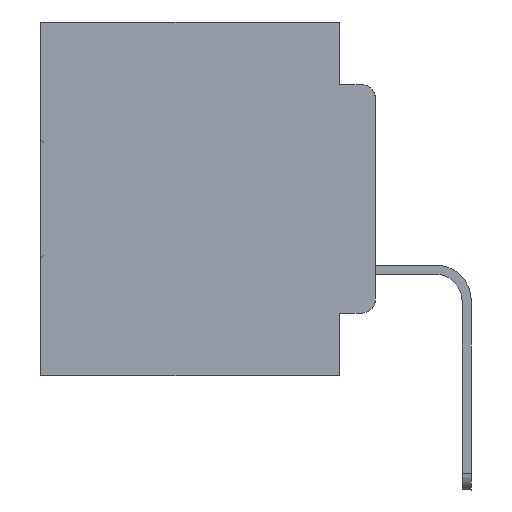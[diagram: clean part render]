
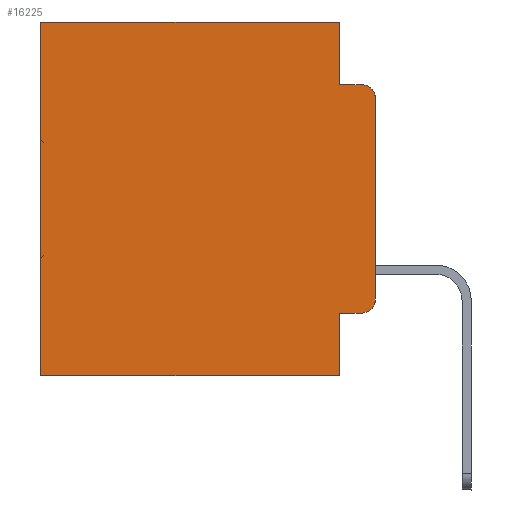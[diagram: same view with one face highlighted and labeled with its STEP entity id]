
A CAD part, left-side view. The second image highlights one B-rep face of the part: STEP entity #16225.
In plain terms, the highlighted planar face has unit normal (-1, 0, 0).
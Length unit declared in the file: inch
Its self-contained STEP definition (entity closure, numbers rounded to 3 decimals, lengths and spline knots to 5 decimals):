
#1254 = CARTESIAN_POINT ( 'NONE',  ( 0.298, 0.473, 0. ) ) ;
#1556 = CIRCLE ( 'NONE', #14137, 0.02 ) ;
#1566 = ORIENTED_EDGE ( 'NONE', *, *, #22731, .F. ) ;
#2893 = CARTESIAN_POINT ( 'NONE',  ( 0.298, 0.051, 0. ) ) ;
#3278 = VERTEX_POINT ( 'NONE', #9668 ) ;
#3466 = DIRECTION ( 'NONE',  ( 0., 0., -1. ) ) ;
#3491 = CARTESIAN_POINT ( 'NONE',  ( 0.298, 0.051, -0.0885 ) ) ;
#3757 = LINE ( 'NONE', #16805, #20361 ) ;
#3810 = VERTEX_POINT ( 'NONE', #14933 ) ;
#4115 = ORIENTED_EDGE ( 'NONE', *, *, #21251, .F. ) ;
#4184 = CARTESIAN_POINT ( 'NONE',  ( 0.298, 0., -0.5 ) ) ;
#4531 = VERTEX_POINT ( 'NONE', #16165 ) ;
#4800 = AXIS2_PLACEMENT_3D ( 'NONE', #22080, #14043, #32391 ) ;
#5301 = LINE ( 'NONE', #13913, #17099 ) ;
#5460 = CARTESIAN_POINT ( 'NONE',  ( 0.298, 0.051, 0. ) ) ;
#5491 = CIRCLE ( 'NONE', #7449, 0.02 ) ;
#7086 = VECTOR ( 'NONE', #21666, 39.37008 ) ;
#7166 = VECTOR ( 'NONE', #11859, 39.37008 ) ;
#7169 = EDGE_CURVE ( 'NONE', #28561, #4531, #31168, .T. ) ;
#7449 = AXIS2_PLACEMENT_3D ( 'NONE', #10569, #18727, #21316 ) ;
#8154 = DIRECTION ( 'NONE',  ( 0., 0., -1. ) ) ;
#8381 = LINE ( 'NONE', #32813, #7166 ) ;
#8784 = CARTESIAN_POINT ( 'NONE',  ( 0.298, 0., -0.3915 ) ) ;
#8978 = PLANE ( 'NONE',  #4800 ) ;
#9665 = LINE ( 'NONE', #15185, #27517 ) ;
#9668 = CARTESIAN_POINT ( 'NONE',  ( 0.298, 0.02, -0.4115 ) ) ;
#10163 = ORIENTED_EDGE ( 'NONE', *, *, #19090, .T. ) ;
#10268 = EDGE_LOOP ( 'NONE', ( #32345, #18417, #1566, #4115, #10540, #31161, #29730, #12635, #10163, #26665 ) ) ;
#10540 = ORIENTED_EDGE ( 'NONE', *, *, #30333, .T. ) ;
#10569 = CARTESIAN_POINT ( 'NONE',  ( 0.298, 0.02, -0.3915 ) ) ;
#11016 = LINE ( 'NONE', #25245, #30481 ) ;
#11797 = CARTESIAN_POINT ( 'NONE',  ( 0.298, 0.02, -0.1085 ) ) ;
#11859 = DIRECTION ( 'NONE',  ( 0., -1., 0. ) ) ;
#12635 = ORIENTED_EDGE ( 'NONE', *, *, #15140, .F. ) ;
#13913 = CARTESIAN_POINT ( 'NONE',  ( 0.298, 0.473, 0. ) ) ;
#13970 = LINE ( 'NONE', #29491, #7086 ) ;
#14043 = DIRECTION ( 'NONE',  ( 1., 0., 0. ) ) ;
#14137 = AXIS2_PLACEMENT_3D ( 'NONE', #11797, #19398, #19717 ) ;
#14933 = CARTESIAN_POINT ( 'NONE',  ( 0.298, 0.02, -0.0885 ) ) ;
#15011 = CARTESIAN_POINT ( 'NONE',  ( 0.298, 0., -0.1085 ) ) ;
#15140 = EDGE_CURVE ( 'NONE', #25811, #28561, #22677, .T. ) ;
#15185 = CARTESIAN_POINT ( 'NONE',  ( 0.298, 0.051, 0. ) ) ;
#16165 = CARTESIAN_POINT ( 'NONE',  ( 0.298, 0.473, -0.5 ) ) ;
#16216 = VERTEX_POINT ( 'NONE', #3491 ) ;
#16225 = ADVANCED_FACE ( 'NONE', ( #18188 ), #8978, .F. ) ;
#16805 = CARTESIAN_POINT ( 'NONE',  ( 0.298, 0., 0. ) ) ;
#17099 = VECTOR ( 'NONE', #3466, 39.37008 ) ;
#17313 = EDGE_CURVE ( 'NONE', #3278, #19053, #5491, .T. ) ;
#17807 = DIRECTION ( 'NONE',  ( 0., 0., -1. ) ) ;
#18188 = FACE_OUTER_BOUND ( 'NONE', #10268, .T. ) ;
#18417 = ORIENTED_EDGE ( 'NONE', *, *, #26735, .T. ) ;
#18727 = DIRECTION ( 'NONE',  ( -1., 0., 0. ) ) ;
#19053 = VERTEX_POINT ( 'NONE', #8784 ) ;
#19090 = EDGE_CURVE ( 'NONE', #25811, #3278, #13970, .T. ) ;
#19275 = DIRECTION ( 'NONE',  ( 0., 1., 0. ) ) ;
#19398 = DIRECTION ( 'NONE',  ( -1., 0., 0. ) ) ;
#19717 = DIRECTION ( 'NONE',  ( 0., 0., -1. ) ) ;
#20361 = VECTOR ( 'NONE', #19275, 39.37008 ) ;
#21251 = EDGE_CURVE ( 'NONE', #23616, #16216, #9665, .T. ) ;
#21316 = DIRECTION ( 'NONE',  ( 0., 0., -1. ) ) ;
#21666 = DIRECTION ( 'NONE',  ( 0., -1., 0. ) ) ;
#22080 = CARTESIAN_POINT ( 'NONE',  ( 0.298, 0., 0. ) ) ;
#22677 = LINE ( 'NONE', #2893, #25951 ) ;
#22731 = EDGE_CURVE ( 'NONE', #16216, #3810, #8381, .T. ) ;
#22779 = VERTEX_POINT ( 'NONE', #15011 ) ;
#23473 = VECTOR ( 'NONE', #30348, 39.37008 ) ;
#23616 = VERTEX_POINT ( 'NONE', #5460 ) ;
#25116 = EDGE_CURVE ( 'NONE', #22779, #19053, #11016, .T. ) ;
#25245 = CARTESIAN_POINT ( 'NONE',  ( 0.298, 0., 0. ) ) ;
#25470 = DIRECTION ( 'NONE',  ( 0., 0., -1. ) ) ;
#25560 = EDGE_CURVE ( 'NONE', #27952, #4531, #5301, .T. ) ;
#25650 = CARTESIAN_POINT ( 'NONE',  ( 0.298, 0.051, -0.4115 ) ) ;
#25811 = VERTEX_POINT ( 'NONE', #25650 ) ;
#25951 = VECTOR ( 'NONE', #8154, 39.37008 ) ;
#26665 = ORIENTED_EDGE ( 'NONE', *, *, #17313, .T. ) ;
#26735 = EDGE_CURVE ( 'NONE', #22779, #3810, #1556, .T. ) ;
#27517 = VECTOR ( 'NONE', #17807, 39.37008 ) ;
#27952 = VERTEX_POINT ( 'NONE', #1254 ) ;
#28561 = VERTEX_POINT ( 'NONE', #29371 ) ;
#29371 = CARTESIAN_POINT ( 'NONE',  ( 0.298, 0.051, -0.5 ) ) ;
#29491 = CARTESIAN_POINT ( 'NONE',  ( 0.298, 0.051, -0.4115 ) ) ;
#29730 = ORIENTED_EDGE ( 'NONE', *, *, #7169, .F. ) ;
#30333 = EDGE_CURVE ( 'NONE', #23616, #27952, #3757, .T. ) ;
#30348 = DIRECTION ( 'NONE',  ( 0., 1., 0. ) ) ;
#30481 = VECTOR ( 'NONE', #25470, 39.37008 ) ;
#31161 = ORIENTED_EDGE ( 'NONE', *, *, #25560, .T. ) ;
#31168 = LINE ( 'NONE', #4184, #23473 ) ;
#32345 = ORIENTED_EDGE ( 'NONE', *, *, #25116, .F. ) ;
#32391 = DIRECTION ( 'NONE',  ( 0., 0., -1. ) ) ;
#32813 = CARTESIAN_POINT ( 'NONE',  ( 0.298, 0.051, -0.0885 ) ) ;
